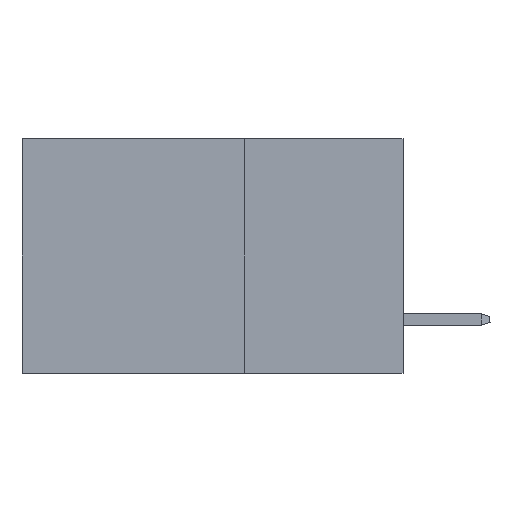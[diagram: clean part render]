
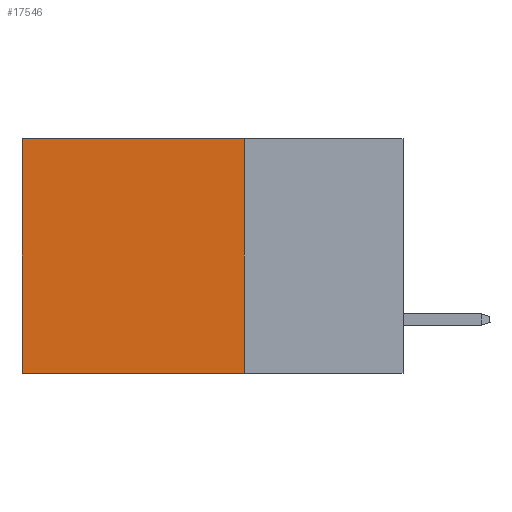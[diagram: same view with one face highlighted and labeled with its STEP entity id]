
A CAD part, left-side view. The second image highlights one B-rep face of the part: STEP entity #17546.
In plain terms, the highlighted planar face has unit normal (-1, 0, 0).
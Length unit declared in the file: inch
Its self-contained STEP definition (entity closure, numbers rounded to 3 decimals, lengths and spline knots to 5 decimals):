
#212 = DIRECTION ( 'NONE',  ( 0., 1., 0. ) ) ;
#1596 = EDGE_CURVE ( 'NONE', #2808, #19624, #10345, .T. ) ;
#2808 = VERTEX_POINT ( 'NONE', #9606 ) ;
#3074 = VECTOR ( 'NONE', #212, 39.37008 ) ;
#4766 = CARTESIAN_POINT ( 'NONE',  ( 0.2875, 0.6, 0. ) ) ;
#5177 = CARTESIAN_POINT ( 'NONE',  ( 0.2875, 0.6, -0.37 ) ) ;
#6132 = EDGE_CURVE ( 'NONE', #19624, #15379, #12986, .T. ) ;
#6207 = CARTESIAN_POINT ( 'NONE',  ( 0.2875, 0.25, -0.37 ) ) ;
#6751 = CARTESIAN_POINT ( 'NONE',  ( 0.2875, 0.25, 0. ) ) ;
#7739 = VECTOR ( 'NONE', #10822, 39.37008 ) ;
#8006 = ORIENTED_EDGE ( 'NONE', *, *, #1596, .F. ) ;
#8036 = CARTESIAN_POINT ( 'NONE',  ( 0.2875, 0.25, -0.37 ) ) ;
#8199 = FACE_OUTER_BOUND ( 'NONE', #18436, .T. ) ;
#8316 = PLANE ( 'NONE',  #13729 ) ;
#8544 = DIRECTION ( 'NONE',  ( 0., 0., -1. ) ) ;
#8610 = EDGE_CURVE ( 'NONE', #2808, #15937, #13702, .T. ) ;
#9606 = CARTESIAN_POINT ( 'NONE',  ( 0.2875, 0.25, 0. ) ) ;
#10078 = ORIENTED_EDGE ( 'NONE', *, *, #8610, .T. ) ;
#10345 = LINE ( 'NONE', #6751, #15060 ) ;
#10785 = CARTESIAN_POINT ( 'NONE',  ( 0.2875, 0.25, 0. ) ) ;
#10822 = DIRECTION ( 'NONE',  ( 0., 1., 0. ) ) ;
#11561 = DIRECTION ( 'NONE',  ( 0., 0., -1. ) ) ;
#12270 = DIRECTION ( 'NONE',  ( 0., 0., -1. ) ) ;
#12986 = LINE ( 'NONE', #6207, #7739 ) ;
#13702 = LINE ( 'NONE', #17504, #3074 ) ;
#13729 = AXIS2_PLACEMENT_3D ( 'NONE', #10785, #20943, #12270 ) ;
#14756 = EDGE_CURVE ( 'NONE', #15937, #15379, #15154, .T. ) ;
#15060 = VECTOR ( 'NONE', #8544, 39.37008 ) ;
#15154 = LINE ( 'NONE', #4766, #15427 ) ;
#15379 = VERTEX_POINT ( 'NONE', #5177 ) ;
#15427 = VECTOR ( 'NONE', #11561, 39.37008 ) ;
#15793 = ORIENTED_EDGE ( 'NONE', *, *, #6132, .F. ) ;
#15937 = VERTEX_POINT ( 'NONE', #17338 ) ;
#17112 = ORIENTED_EDGE ( 'NONE', *, *, #14756, .T. ) ;
#17338 = CARTESIAN_POINT ( 'NONE',  ( 0.2875, 0.6, 0. ) ) ;
#17504 = CARTESIAN_POINT ( 'NONE',  ( 0.2875, 0.25, 0. ) ) ;
#17546 = ADVANCED_FACE ( 'NONE', ( #8199 ), #8316, .F. ) ;
#18436 = EDGE_LOOP ( 'NONE', ( #17112, #15793, #8006, #10078 ) ) ;
#19624 = VERTEX_POINT ( 'NONE', #8036 ) ;
#20943 = DIRECTION ( 'NONE',  ( 1., 0., 0. ) ) ;
